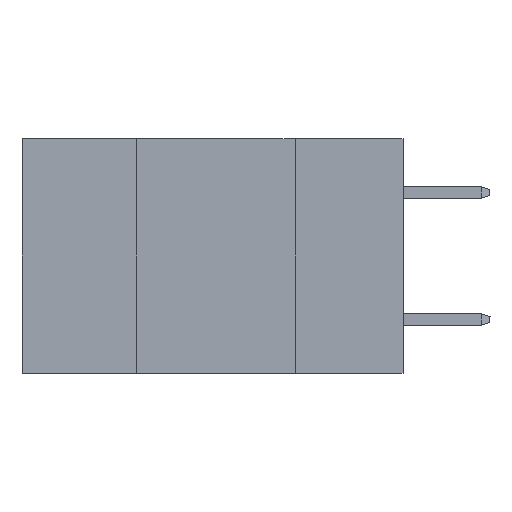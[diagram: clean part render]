
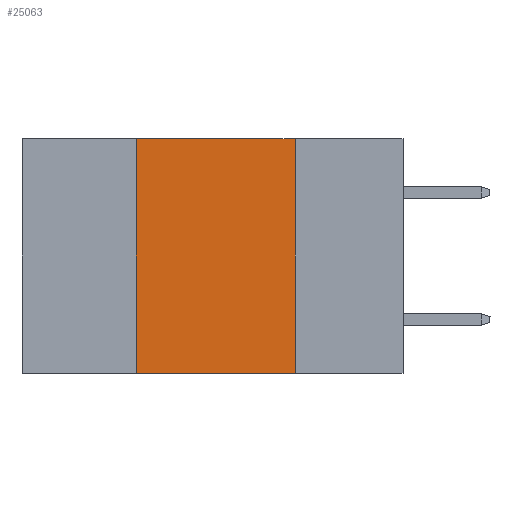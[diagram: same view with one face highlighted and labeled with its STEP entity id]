
A CAD part, left-side view. The second image highlights one B-rep face of the part: STEP entity #25063.
In plain terms, the highlighted planar face has unit normal (-1, 0, 0).
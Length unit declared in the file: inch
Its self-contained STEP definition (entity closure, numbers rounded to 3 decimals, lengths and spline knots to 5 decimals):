
#1183 = DIRECTION ( 'NONE',  ( 0., -1., 0. ) ) ;
#2025 = ORIENTED_EDGE ( 'NONE', *, *, #24761, .F. ) ;
#2095 = LINE ( 'NONE', #2347, #2607 ) ;
#2172 = CARTESIAN_POINT ( 'NONE',  ( 0., 0.6, -0.37 ) ) ;
#2247 = LINE ( 'NONE', #10015, #17231 ) ;
#2343 = DIRECTION ( 'NONE',  ( 1., 0., 0. ) ) ;
#2347 = CARTESIAN_POINT ( 'NONE',  ( 0., 0.17, 0. ) ) ;
#2607 = VECTOR ( 'NONE', #20046, 39.37008 ) ;
#3000 = VERTEX_POINT ( 'NONE', #12437 ) ;
#3022 = EDGE_LOOP ( 'NONE', ( #22318, #2025, #13408, #9483 ) ) ;
#4370 = VERTEX_POINT ( 'NONE', #16028 ) ;
#6814 = VERTEX_POINT ( 'NONE', #23968 ) ;
#7280 = LINE ( 'NONE', #19415, #11315 ) ;
#9483 = ORIENTED_EDGE ( 'NONE', *, *, #14011, .T. ) ;
#9638 = VECTOR ( 'NONE', #16211, 39.37008 ) ;
#10015 = CARTESIAN_POINT ( 'NONE',  ( 0., 0.42, 0. ) ) ;
#11315 = VECTOR ( 'NONE', #1183, 39.37008 ) ;
#12437 = CARTESIAN_POINT ( 'NONE',  ( 0., 0.42, -0.37 ) ) ;
#13408 = ORIENTED_EDGE ( 'NONE', *, *, #17481, .F. ) ;
#14011 = EDGE_CURVE ( 'NONE', #3000, #6814, #24072, .T. ) ;
#16024 = CARTESIAN_POINT ( 'NONE',  ( 0., 0.42, 0. ) ) ;
#16028 = CARTESIAN_POINT ( 'NONE',  ( 0., 0.17, 0. ) ) ;
#16211 = DIRECTION ( 'NONE',  ( 0., -1., 0. ) ) ;
#17231 = VECTOR ( 'NONE', #22158, 39.37008 ) ;
#17481 = EDGE_CURVE ( 'NONE', #3000, #19601, #2247, .T. ) ;
#18577 = EDGE_CURVE ( 'NONE', #4370, #6814, #2095, .T. ) ;
#19415 = CARTESIAN_POINT ( 'NONE',  ( 0., 0.6, 0. ) ) ;
#19601 = VERTEX_POINT ( 'NONE', #16024 ) ;
#20046 = DIRECTION ( 'NONE',  ( 0., 0., -1. ) ) ;
#20553 = DIRECTION ( 'NONE',  ( 0., 0., -1. ) ) ;
#22158 = DIRECTION ( 'NONE',  ( 0., 0., 1. ) ) ;
#22173 = AXIS2_PLACEMENT_3D ( 'NONE', #22261, #2343, #20553 ) ;
#22261 = CARTESIAN_POINT ( 'NONE',  ( 0., 0.6, 0. ) ) ;
#22318 = ORIENTED_EDGE ( 'NONE', *, *, #18577, .F. ) ;
#22392 = FACE_OUTER_BOUND ( 'NONE', #3022, .T. ) ;
#23968 = CARTESIAN_POINT ( 'NONE',  ( 0., 0.17, -0.37 ) ) ;
#24072 = LINE ( 'NONE', #2172, #9638 ) ;
#24645 = PLANE ( 'NONE',  #22173 ) ;
#24761 = EDGE_CURVE ( 'NONE', #19601, #4370, #7280, .T. ) ;
#25063 = ADVANCED_FACE ( 'NONE', ( #22392 ), #24645, .F. ) ;
